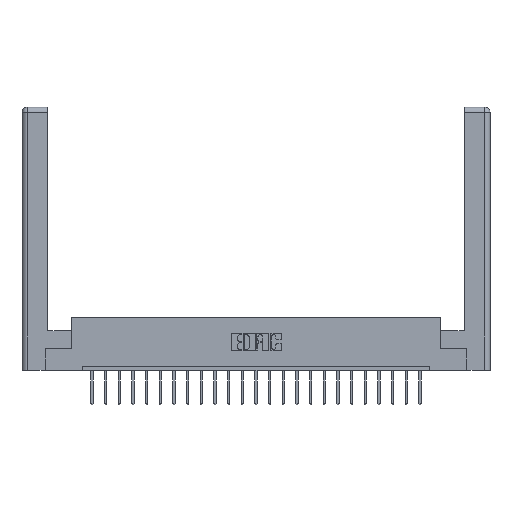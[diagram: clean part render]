
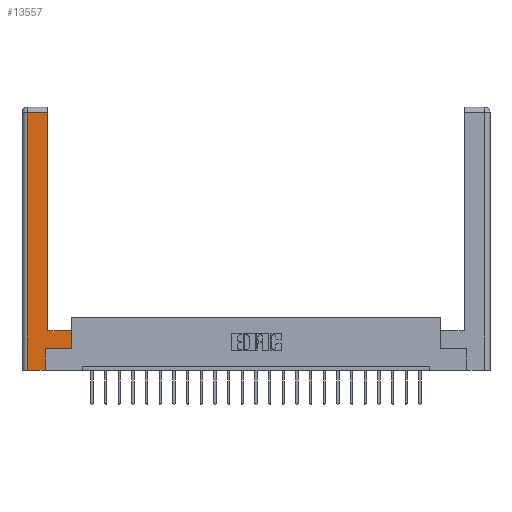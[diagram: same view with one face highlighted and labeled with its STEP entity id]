
A CAD part, top view. The second image highlights one B-rep face of the part: STEP entity #13557.
In plain terms, the highlighted planar face has unit normal (0, 0, 1).
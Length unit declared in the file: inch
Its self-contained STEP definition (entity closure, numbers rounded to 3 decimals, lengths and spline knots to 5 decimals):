
#241 = VERTEX_POINT ( 'NONE', #22925 ) ;
#386 = DIRECTION ( 'NONE',  ( -1., 0., 0. ) ) ;
#391 = EDGE_CURVE ( 'NONE', #22604, #21612, #12377, .T. ) ;
#472 = DIRECTION ( 'NONE',  ( 0., 1., 0. ) ) ;
#535 = CARTESIAN_POINT ( 'NONE',  ( 0.0615, 2.94, 0. ) ) ;
#947 = VECTOR ( 'NONE', #18462, 39.37008 ) ;
#1442 = CARTESIAN_POINT ( 'NONE',  ( 0.295, 2.94, 0. ) ) ;
#1669 = VERTEX_POINT ( 'NONE', #19345 ) ;
#1894 = LINE ( 'NONE', #11672, #15993 ) ;
#1946 = DIRECTION ( 'NONE',  ( 0., -1., 0. ) ) ;
#2210 = ORIENTED_EDGE ( 'NONE', *, *, #22071, .T. ) ;
#2796 = CARTESIAN_POINT ( 'NONE',  ( 0.565, 0.245, 0. ) ) ;
#2904 = EDGE_CURVE ( 'NONE', #4758, #18548, #9471, .T. ) ;
#3609 = EDGE_CURVE ( 'NONE', #12647, #6255, #15354, .T. ) ;
#3794 = LINE ( 'NONE', #9349, #22454 ) ;
#4181 = DIRECTION ( 'NONE',  ( 0., 0., -1. ) ) ;
#4392 = CARTESIAN_POINT ( 'NONE',  ( 0.265, 0.245, 0. ) ) ;
#4681 = VECTOR ( 'NONE', #472, 39.37008 ) ;
#4758 = VERTEX_POINT ( 'NONE', #7182 ) ;
#5187 = ORIENTED_EDGE ( 'NONE', *, *, #3609, .T. ) ;
#5244 = CARTESIAN_POINT ( 'NONE',  ( 0.565, 0.45, 0. ) ) ;
#5395 = ORIENTED_EDGE ( 'NONE', *, *, #2904, .T. ) ;
#5429 = EDGE_CURVE ( 'NONE', #18548, #241, #1894, .T. ) ;
#6255 = VERTEX_POINT ( 'NONE', #14770 ) ;
#6863 = LINE ( 'NONE', #15078, #15885 ) ;
#7182 = CARTESIAN_POINT ( 'NONE',  ( 0.565, 0.245, 0. ) ) ;
#7661 = VECTOR ( 'NONE', #10374, 39.37008 ) ;
#7885 = AXIS2_PLACEMENT_3D ( 'NONE', #14996, #4181, #18618 ) ;
#9349 = CARTESIAN_POINT ( 'NONE',  ( 0.0615, 0., 0. ) ) ;
#9471 = LINE ( 'NONE', #11437, #4681 ) ;
#10374 = DIRECTION ( 'NONE',  ( 1., 0., 0. ) ) ;
#11160 = EDGE_CURVE ( 'NONE', #1669, #4758, #17567, .T. ) ;
#11207 = CARTESIAN_POINT ( 'NONE',  ( 0.0615, 2.94, 0. ) ) ;
#11408 = DIRECTION ( 'NONE',  ( 0., 1., 0. ) ) ;
#11437 = CARTESIAN_POINT ( 'NONE',  ( 0.565, 0.45, 0. ) ) ;
#11489 = ORIENTED_EDGE ( 'NONE', *, *, #391, .T. ) ;
#11672 = CARTESIAN_POINT ( 'NONE',  ( 0.295, 0.45, 0. ) ) ;
#12377 = LINE ( 'NONE', #11207, #18311 ) ;
#12647 = VERTEX_POINT ( 'NONE', #18028 ) ;
#13042 = FACE_OUTER_BOUND ( 'NONE', #20307, .T. ) ;
#13324 = PLANE ( 'NONE',  #7885 ) ;
#13494 = EDGE_CURVE ( 'NONE', #241, #22604, #6863, .T. ) ;
#13557 = ADVANCED_FACE ( 'NONE', ( #13042 ), #13324, .F. ) ;
#13864 = VECTOR ( 'NONE', #11408, 39.37008 ) ;
#14171 = EDGE_CURVE ( 'NONE', #6255, #1669, #23239, .T. ) ;
#14770 = CARTESIAN_POINT ( 'NONE',  ( 0.265, 0., 0. ) ) ;
#14837 = DIRECTION ( 'NONE',  ( 0., 1., 0. ) ) ;
#14996 = CARTESIAN_POINT ( 'NONE',  ( 0., 0., 0. ) ) ;
#15078 = CARTESIAN_POINT ( 'NONE',  ( 0.295, 3., 0. ) ) ;
#15354 = LINE ( 'NONE', #19910, #947 ) ;
#15885 = VECTOR ( 'NONE', #14837, 39.37008 ) ;
#15993 = VECTOR ( 'NONE', #17121, 39.37008 ) ;
#17121 = DIRECTION ( 'NONE',  ( -1., 0., 0. ) ) ;
#17386 = ORIENTED_EDGE ( 'NONE', *, *, #14171, .T. ) ;
#17567 = LINE ( 'NONE', #2796, #7661 ) ;
#18028 = CARTESIAN_POINT ( 'NONE',  ( 0.0615, 0., 0. ) ) ;
#18297 = ORIENTED_EDGE ( 'NONE', *, *, #11160, .T. ) ;
#18311 = VECTOR ( 'NONE', #386, 39.37008 ) ;
#18462 = DIRECTION ( 'NONE',  ( 1., 0., 0. ) ) ;
#18548 = VERTEX_POINT ( 'NONE', #5244 ) ;
#18618 = DIRECTION ( 'NONE',  ( -1., 0., 0. ) ) ;
#19345 = CARTESIAN_POINT ( 'NONE',  ( 0.265, 0.245, 0. ) ) ;
#19910 = CARTESIAN_POINT ( 'NONE',  ( 0.265, 0., 0. ) ) ;
#20307 = EDGE_LOOP ( 'NONE', ( #22965, #11489, #2210, #5187, #17386, #18297, #5395, #20906 ) ) ;
#20906 = ORIENTED_EDGE ( 'NONE', *, *, #5429, .T. ) ;
#21612 = VERTEX_POINT ( 'NONE', #535 ) ;
#22071 = EDGE_CURVE ( 'NONE', #21612, #12647, #3794, .T. ) ;
#22454 = VECTOR ( 'NONE', #1946, 39.37008 ) ;
#22604 = VERTEX_POINT ( 'NONE', #1442 ) ;
#22925 = CARTESIAN_POINT ( 'NONE',  ( 0.295, 0.45, 0. ) ) ;
#22965 = ORIENTED_EDGE ( 'NONE', *, *, #13494, .T. ) ;
#23239 = LINE ( 'NONE', #4392, #13864 ) ;
